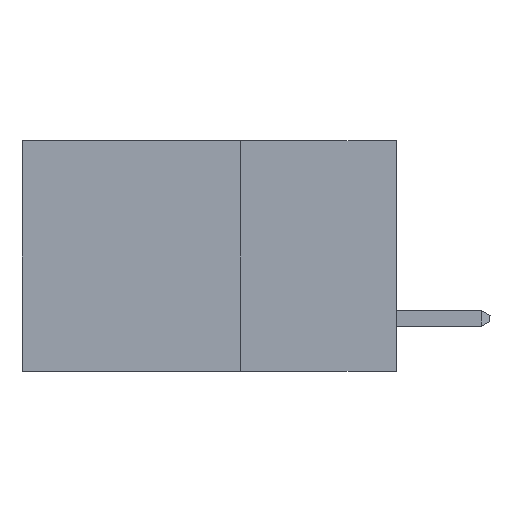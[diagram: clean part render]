
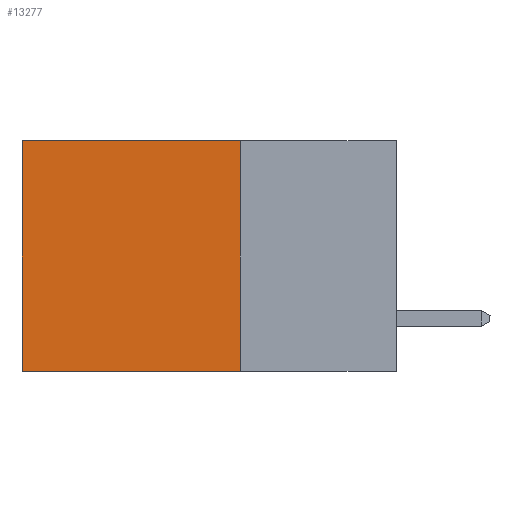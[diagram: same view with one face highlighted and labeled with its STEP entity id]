
A CAD part, left-side view. The second image highlights one B-rep face of the part: STEP entity #13277.
In plain terms, the highlighted planar face has unit normal (-1, 0, 0).
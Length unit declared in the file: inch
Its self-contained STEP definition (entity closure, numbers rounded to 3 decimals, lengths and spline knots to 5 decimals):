
#1032 = DIRECTION ( 'NONE',  ( 0., 1., 0. ) ) ;
#1612 = FACE_OUTER_BOUND ( 'NONE', #18010, .T. ) ;
#1745 = CARTESIAN_POINT ( 'NONE',  ( 0.2615, 0.25, 0. ) ) ;
#2213 = DIRECTION ( 'NONE',  ( 0., 1., 0. ) ) ;
#2295 = CARTESIAN_POINT ( 'NONE',  ( 0.2615, 0.25, -0.37 ) ) ;
#2753 = LINE ( 'NONE', #11187, #12567 ) ;
#2791 = VERTEX_POINT ( 'NONE', #9861 ) ;
#2978 = DIRECTION ( 'NONE',  ( 0., 0., -1. ) ) ;
#3011 = DIRECTION ( 'NONE',  ( 1., 0., 0. ) ) ;
#3149 = PLANE ( 'NONE',  #17577 ) ;
#3255 = CARTESIAN_POINT ( 'NONE',  ( 0.2615, 0.25, -0.37 ) ) ;
#3742 = DIRECTION ( 'NONE',  ( 0., 0., -1. ) ) ;
#4331 = DIRECTION ( 'NONE',  ( 0., 0., -1. ) ) ;
#4599 = LINE ( 'NONE', #8009, #22675 ) ;
#4607 = LINE ( 'NONE', #2295, #9009 ) ;
#5152 = VERTEX_POINT ( 'NONE', #15583 ) ;
#6733 = EDGE_CURVE ( 'NONE', #5152, #2791, #4607, .T. ) ;
#7599 = VECTOR ( 'NONE', #1032, 39.37008 ) ;
#8009 = CARTESIAN_POINT ( 'NONE',  ( 0.2615, 0.6, -0.37 ) ) ;
#8500 = CARTESIAN_POINT ( 'NONE',  ( 0.2615, 0.6, 0. ) ) ;
#9009 = VECTOR ( 'NONE', #2213, 39.37008 ) ;
#9861 = CARTESIAN_POINT ( 'NONE',  ( 0.2615, 0.6, -0.37 ) ) ;
#11187 = CARTESIAN_POINT ( 'NONE',  ( 0.2615, 0.25, -0.37 ) ) ;
#12251 = ORIENTED_EDGE ( 'NONE', *, *, #16665, .F. ) ;
#12567 = VECTOR ( 'NONE', #3742, 39.37008 ) ;
#12712 = VERTEX_POINT ( 'NONE', #8500 ) ;
#13277 = ADVANCED_FACE ( 'NONE', ( #1612 ), #3149, .F. ) ;
#15583 = CARTESIAN_POINT ( 'NONE',  ( 0.2615, 0.25, -0.37 ) ) ;
#16665 = EDGE_CURVE ( 'NONE', #20534, #5152, #2753, .T. ) ;
#17577 = AXIS2_PLACEMENT_3D ( 'NONE', #3255, #3011, #2978 ) ;
#18010 = EDGE_LOOP ( 'NONE', ( #18523, #19824, #12251, #19703 ) ) ;
#18311 = LINE ( 'NONE', #22792, #7599 ) ;
#18523 = ORIENTED_EDGE ( 'NONE', *, *, #20116, .T. ) ;
#19532 = EDGE_CURVE ( 'NONE', #20534, #12712, #18311, .T. ) ;
#19703 = ORIENTED_EDGE ( 'NONE', *, *, #19532, .T. ) ;
#19824 = ORIENTED_EDGE ( 'NONE', *, *, #6733, .F. ) ;
#20116 = EDGE_CURVE ( 'NONE', #12712, #2791, #4599, .T. ) ;
#20534 = VERTEX_POINT ( 'NONE', #1745 ) ;
#22675 = VECTOR ( 'NONE', #4331, 39.37008 ) ;
#22792 = CARTESIAN_POINT ( 'NONE',  ( 0.2615, 0.25, 0. ) ) ;
